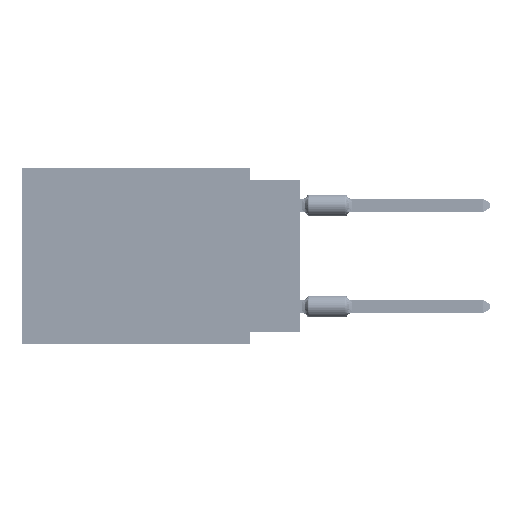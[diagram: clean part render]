
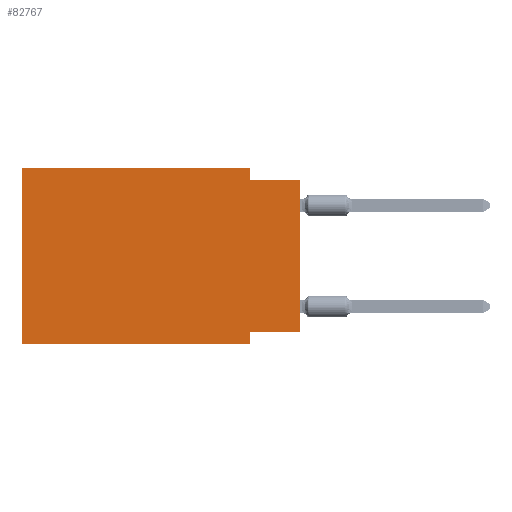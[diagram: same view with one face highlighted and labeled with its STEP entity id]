
A CAD part, left-side view. The second image highlights one B-rep face of the part: STEP entity #82767.
In plain terms, the highlighted planar face has unit normal (-1, 0, 0).
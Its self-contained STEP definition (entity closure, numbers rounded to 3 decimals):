
#2976 = VECTOR ( 'NONE', #69138, 1000. ) ;
#3169 = DIRECTION ( 'NONE',  ( 0., 0., -1. ) ) ;
#6181 = LINE ( 'NONE', #20098, #87160 ) ;
#7385 = VECTOR ( 'NONE', #67912, 1000. ) ;
#10175 = EDGE_CURVE ( 'NONE', #83371, #15731, #85004, .T. ) ;
#10199 = ORIENTED_EDGE ( 'NONE', *, *, #19633, .F. ) ;
#10504 = VECTOR ( 'NONE', #76206, 1000. ) ;
#12002 = EDGE_CURVE ( 'NONE', #95721, #57878, #20067, .T. ) ;
#12380 = ORIENTED_EDGE ( 'NONE', *, *, #87383, .F. ) ;
#14970 = DIRECTION ( 'NONE',  ( 0., -1., 0. ) ) ;
#15731 = VERTEX_POINT ( 'NONE', #73043 ) ;
#18060 = CARTESIAN_POINT ( 'NONE',  ( 0., 13.97, -8.89 ) ) ;
#19633 = EDGE_CURVE ( 'NONE', #43709, #31348, #99259, .T. ) ;
#20067 = LINE ( 'NONE', #27792, #74305 ) ;
#20098 = CARTESIAN_POINT ( 'NONE',  ( 0., 13.97, 0. ) ) ;
#20188 = ORIENTED_EDGE ( 'NONE', *, *, #12002, .F. ) ;
#23208 = CARTESIAN_POINT ( 'NONE',  ( 0., 13.97, -8.89 ) ) ;
#24161 = VERTEX_POINT ( 'NONE', #49297 ) ;
#25485 = CARTESIAN_POINT ( 'NONE',  ( 0., 2.54, -0.635 ) ) ;
#26315 = CARTESIAN_POINT ( 'NONE',  ( 0., 0., -8.255 ) ) ;
#27792 = CARTESIAN_POINT ( 'NONE',  ( 0., 2.54, -8.89 ) ) ;
#28151 = AXIS2_PLACEMENT_3D ( 'NONE', #62963, #94291, #85553 ) ;
#29084 = EDGE_CURVE ( 'NONE', #43709, #57878, #53030, .T. ) ;
#29337 = DIRECTION ( 'NONE',  ( 0., -1., 0. ) ) ;
#29893 = CARTESIAN_POINT ( 'NONE',  ( 0., 2.54, -8.89 ) ) ;
#31348 = VERTEX_POINT ( 'NONE', #99270 ) ;
#37292 = LINE ( 'NONE', #68644, #2976 ) ;
#43709 = VERTEX_POINT ( 'NONE', #18060 ) ;
#44865 = LINE ( 'NONE', #54628, #10504 ) ;
#45384 = VECTOR ( 'NONE', #14970, 1000. ) ;
#45704 = CARTESIAN_POINT ( 'NONE',  ( 0., 2.54, -8.255 ) ) ;
#45801 = CARTESIAN_POINT ( 'NONE',  ( 0., 13.97, 0. ) ) ;
#49297 = CARTESIAN_POINT ( 'NONE',  ( 0., 2.54, 0. ) ) ;
#53030 = LINE ( 'NONE', #23208, #45384 ) ;
#53850 = VECTOR ( 'NONE', #54196, 1000. ) ;
#54196 = DIRECTION ( 'NONE',  ( 0., 0., 1. ) ) ;
#54528 = EDGE_CURVE ( 'NONE', #69037, #15731, #37292, .T. ) ;
#54628 = CARTESIAN_POINT ( 'NONE',  ( 0., 0., -8.255 ) ) ;
#57668 = LINE ( 'NONE', #96208, #100745 ) ;
#57878 = VERTEX_POINT ( 'NONE', #29893 ) ;
#62963 = CARTESIAN_POINT ( 'NONE',  ( 0., 13.97, 0. ) ) ;
#63477 = PLANE ( 'NONE',  #28151 ) ;
#63548 = ORIENTED_EDGE ( 'NONE', *, *, #54528, .F. ) ;
#66724 = EDGE_CURVE ( 'NONE', #31348, #24161, #6181, .T. ) ;
#67846 = DIRECTION ( 'NONE',  ( 0., 0., -1. ) ) ;
#67912 = DIRECTION ( 'NONE',  ( 0., 0., 1. ) ) ;
#68644 = CARTESIAN_POINT ( 'NONE',  ( 0., 0., -0.635 ) ) ;
#69037 = VERTEX_POINT ( 'NONE', #25485 ) ;
#69138 = DIRECTION ( 'NONE',  ( 0., -1., 0. ) ) ;
#73043 = CARTESIAN_POINT ( 'NONE',  ( 0., 0., -0.635 ) ) ;
#74305 = VECTOR ( 'NONE', #67846, 1000. ) ;
#76206 = DIRECTION ( 'NONE',  ( 0., 1., 0. ) ) ;
#76563 = ORIENTED_EDGE ( 'NONE', *, *, #29084, .T. ) ;
#78353 = FACE_OUTER_BOUND ( 'NONE', #78577, .T. ) ;
#78577 = EDGE_LOOP ( 'NONE', ( #79430, #63548, #12380, #95554, #10199, #76563, #20188, #87910 ) ) ;
#79430 = ORIENTED_EDGE ( 'NONE', *, *, #10175, .T. ) ;
#82767 = ADVANCED_FACE ( 'NONE', ( #78353 ), #63477, .F. ) ;
#83371 = VERTEX_POINT ( 'NONE', #26315 ) ;
#85004 = LINE ( 'NONE', #93226, #53850 ) ;
#85553 = DIRECTION ( 'NONE',  ( 0., 0., -1. ) ) ;
#87160 = VECTOR ( 'NONE', #29337, 1000. ) ;
#87383 = EDGE_CURVE ( 'NONE', #24161, #69037, #57668, .T. ) ;
#87910 = ORIENTED_EDGE ( 'NONE', *, *, #100068, .F. ) ;
#93226 = CARTESIAN_POINT ( 'NONE',  ( 0., 0., 0. ) ) ;
#94291 = DIRECTION ( 'NONE',  ( 1., 0., 0. ) ) ;
#95554 = ORIENTED_EDGE ( 'NONE', *, *, #66724, .F. ) ;
#95721 = VERTEX_POINT ( 'NONE', #45704 ) ;
#96208 = CARTESIAN_POINT ( 'NONE',  ( 0., 2.54, 0. ) ) ;
#99259 = LINE ( 'NONE', #45801, #7385 ) ;
#99270 = CARTESIAN_POINT ( 'NONE',  ( 0., 13.97, 0. ) ) ;
#100068 = EDGE_CURVE ( 'NONE', #83371, #95721, #44865, .T. ) ;
#100745 = VECTOR ( 'NONE', #3169, 1000. ) ;
